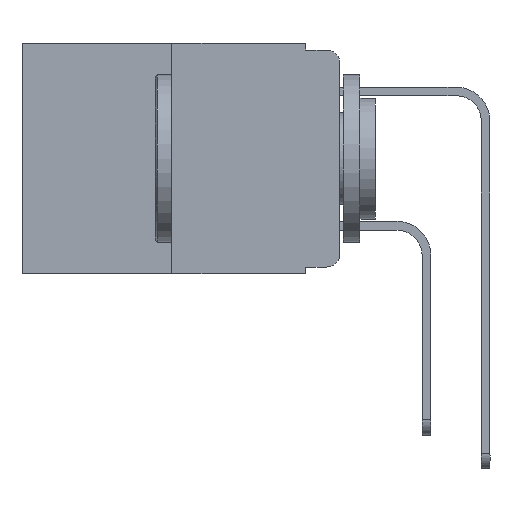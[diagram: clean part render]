
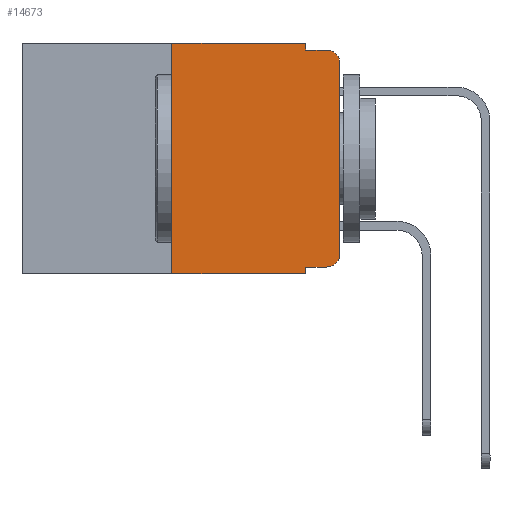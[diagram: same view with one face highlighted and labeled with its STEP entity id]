
A CAD part, left-side view. The second image highlights one B-rep face of the part: STEP entity #14673.
In plain terms, the highlighted planar face has unit normal (-1, 0, 0).
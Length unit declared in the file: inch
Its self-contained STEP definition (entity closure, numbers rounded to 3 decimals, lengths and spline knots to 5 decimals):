
#747 = EDGE_LOOP ( 'NONE', ( #6104, #9186, #21102, #3877, #16686, #4992, #22662, #22422, #16474, #21798 ) ) ;
#819 = CARTESIAN_POINT ( 'NONE',  ( 0., 0.02, -0.333 ) ) ;
#1035 = LINE ( 'NONE', #10123, #16368 ) ;
#1134 = LINE ( 'NONE', #13473, #11167 ) ;
#1297 = VERTEX_POINT ( 'NONE', #819 ) ;
#1370 = DIRECTION ( 'NONE',  ( 0., 0., 1. ) ) ;
#1740 = VERTEX_POINT ( 'NONE', #12271 ) ;
#1849 = EDGE_CURVE ( 'NONE', #9218, #17033, #15994, .T. ) ;
#2190 = VERTEX_POINT ( 'NONE', #7225 ) ;
#2826 = AXIS2_PLACEMENT_3D ( 'NONE', #13674, #4355, #18803 ) ;
#3330 = DIRECTION ( 'NONE',  ( 1., 0., 0. ) ) ;
#3449 = CARTESIAN_POINT ( 'NONE',  ( 0., 0.02, -0.313 ) ) ;
#3877 = ORIENTED_EDGE ( 'NONE', *, *, #21844, .F. ) ;
#4314 = VECTOR ( 'NONE', #14882, 39.37008 ) ;
#4355 = DIRECTION ( 'NONE',  ( -1., 0., 0. ) ) ;
#4837 = CARTESIAN_POINT ( 'NONE',  ( 0., 0.051, -0.01 ) ) ;
#4992 = ORIENTED_EDGE ( 'NONE', *, *, #20703, .F. ) ;
#5070 = PLANE ( 'NONE',  #19550 ) ;
#5101 = CARTESIAN_POINT ( 'NONE',  ( 0., 0.051, -0.333 ) ) ;
#5322 = DIRECTION ( 'NONE',  ( 0., -1., 0. ) ) ;
#5352 = CARTESIAN_POINT ( 'NONE',  ( 0., 0.25, 0. ) ) ;
#5531 = CARTESIAN_POINT ( 'NONE',  ( 0., 0.25, -0.343 ) ) ;
#5594 = LINE ( 'NONE', #5352, #12243 ) ;
#5848 = DIRECTION ( 'NONE',  ( 0., -1., 0. ) ) ;
#6104 = ORIENTED_EDGE ( 'NONE', *, *, #20100, .T. ) ;
#6256 = CARTESIAN_POINT ( 'NONE',  ( 0., 0.473, 0. ) ) ;
#6813 = EDGE_CURVE ( 'NONE', #8350, #17033, #7634, .T. ) ;
#6998 = CARTESIAN_POINT ( 'NONE',  ( 0., 0., -0.313 ) ) ;
#7078 = VECTOR ( 'NONE', #19052, 39.37008 ) ;
#7225 = CARTESIAN_POINT ( 'NONE',  ( 0., 0.25, 0. ) ) ;
#7634 = LINE ( 'NONE', #14980, #14153 ) ;
#7774 = LINE ( 'NONE', #6256, #4314 ) ;
#8088 = VERTEX_POINT ( 'NONE', #15208 ) ;
#8350 = VERTEX_POINT ( 'NONE', #19720 ) ;
#9186 = ORIENTED_EDGE ( 'NONE', *, *, #9823, .T. ) ;
#9218 = VERTEX_POINT ( 'NONE', #5531 ) ;
#9823 = EDGE_CURVE ( 'NONE', #1740, #18312, #13950, .T. ) ;
#10123 = CARTESIAN_POINT ( 'NONE',  ( 0., 0., 0. ) ) ;
#10225 = DIRECTION ( 'NONE',  ( 0., 0., -1. ) ) ;
#10294 = VERTEX_POINT ( 'NONE', #18892 ) ;
#10339 = FACE_OUTER_BOUND ( 'NONE', #747, .T. ) ;
#11167 = VECTOR ( 'NONE', #13238, 39.37008 ) ;
#11385 = VECTOR ( 'NONE', #5848, 39.37008 ) ;
#11926 = VERTEX_POINT ( 'NONE', #6998 ) ;
#12243 = VECTOR ( 'NONE', #16202, 39.37008 ) ;
#12271 = CARTESIAN_POINT ( 'NONE',  ( 0., 0., -0.03 ) ) ;
#13238 = DIRECTION ( 'NONE',  ( 0., 0., -1. ) ) ;
#13473 = CARTESIAN_POINT ( 'NONE',  ( 0., 0.051, 0. ) ) ;
#13674 = CARTESIAN_POINT ( 'NONE',  ( 0., 0.02, -0.03 ) ) ;
#13950 = CIRCLE ( 'NONE', #2826, 0.02 ) ;
#14153 = VECTOR ( 'NONE', #18593, 39.37008 ) ;
#14273 = EDGE_CURVE ( 'NONE', #8350, #1297, #20855, .T. ) ;
#14673 = ADVANCED_FACE ( 'NONE', ( #10339 ), #5070, .F. ) ;
#14882 = DIRECTION ( 'NONE',  ( 0., -1., 0. ) ) ;
#14980 = CARTESIAN_POINT ( 'NONE',  ( 0., 0.051, 0. ) ) ;
#15208 = CARTESIAN_POINT ( 'NONE',  ( 0., 0.051, -0.01 ) ) ;
#15638 = CARTESIAN_POINT ( 'NONE',  ( 0., 0.051, -0.343 ) ) ;
#15994 = LINE ( 'NONE', #16701, #11385 ) ;
#16202 = DIRECTION ( 'NONE',  ( 0., 0., 1. ) ) ;
#16368 = VECTOR ( 'NONE', #1370, 39.37008 ) ;
#16377 = EDGE_CURVE ( 'NONE', #2190, #10294, #7774, .T. ) ;
#16474 = ORIENTED_EDGE ( 'NONE', *, *, #14273, .T. ) ;
#16686 = ORIENTED_EDGE ( 'NONE', *, *, #16377, .F. ) ;
#16701 = CARTESIAN_POINT ( 'NONE',  ( 0., 0.473, -0.343 ) ) ;
#17033 = VERTEX_POINT ( 'NONE', #15638 ) ;
#17127 = CIRCLE ( 'NONE', #18973, 0.02 ) ;
#17206 = LINE ( 'NONE', #4837, #7078 ) ;
#17561 = CARTESIAN_POINT ( 'NONE',  ( 0., 0.473, 0. ) ) ;
#17567 = DIRECTION ( 'NONE',  ( 0., 0., -1. ) ) ;
#18312 = VERTEX_POINT ( 'NONE', #21783 ) ;
#18593 = DIRECTION ( 'NONE',  ( 0., 0., -1. ) ) ;
#18803 = DIRECTION ( 'NONE',  ( 0., 0., -1. ) ) ;
#18892 = CARTESIAN_POINT ( 'NONE',  ( 0., 0.051, 0. ) ) ;
#18973 = AXIS2_PLACEMENT_3D ( 'NONE', #3449, #19520, #17567 ) ;
#19052 = DIRECTION ( 'NONE',  ( 0., -1., 0. ) ) ;
#19172 = VECTOR ( 'NONE', #5322, 39.37008 ) ;
#19520 = DIRECTION ( 'NONE',  ( -1., 0., 0. ) ) ;
#19550 = AXIS2_PLACEMENT_3D ( 'NONE', #17561, #3330, #10225 ) ;
#19720 = CARTESIAN_POINT ( 'NONE',  ( 0., 0.051, -0.333 ) ) ;
#20100 = EDGE_CURVE ( 'NONE', #11926, #1740, #1035, .T. ) ;
#20703 = EDGE_CURVE ( 'NONE', #9218, #2190, #5594, .T. ) ;
#20855 = LINE ( 'NONE', #5101, #19172 ) ;
#21102 = ORIENTED_EDGE ( 'NONE', *, *, #21938, .F. ) ;
#21600 = EDGE_CURVE ( 'NONE', #1297, #11926, #17127, .T. ) ;
#21783 = CARTESIAN_POINT ( 'NONE',  ( 0., 0.02, -0.01 ) ) ;
#21798 = ORIENTED_EDGE ( 'NONE', *, *, #21600, .T. ) ;
#21844 = EDGE_CURVE ( 'NONE', #10294, #8088, #1134, .T. ) ;
#21938 = EDGE_CURVE ( 'NONE', #8088, #18312, #17206, .T. ) ;
#22422 = ORIENTED_EDGE ( 'NONE', *, *, #6813, .F. ) ;
#22662 = ORIENTED_EDGE ( 'NONE', *, *, #1849, .T. ) ;
